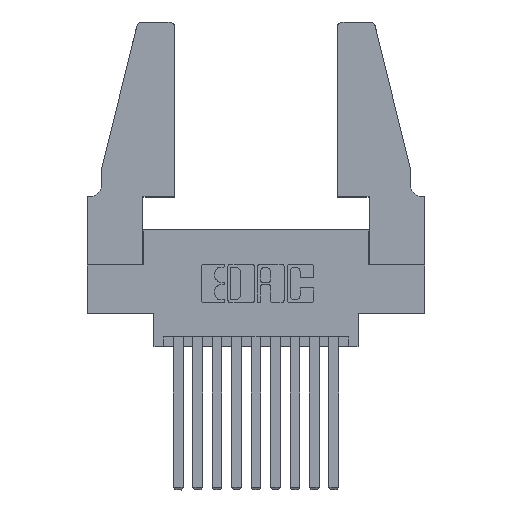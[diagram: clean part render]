
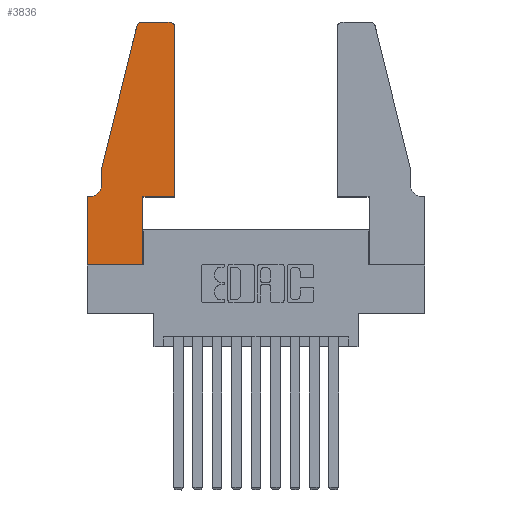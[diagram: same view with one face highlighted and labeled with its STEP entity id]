
A CAD part, top view. The second image highlights one B-rep face of the part: STEP entity #3836.
In plain terms, the highlighted planar face has unit normal (0, 0, 1).
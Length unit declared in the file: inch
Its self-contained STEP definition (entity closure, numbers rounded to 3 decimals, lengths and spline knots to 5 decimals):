
#142 = ORIENTED_EDGE ( 'NONE', *, *, #3117, .T. ) ;
#378 = CARTESIAN_POINT ( 'NONE',  ( 0.0755, 0.5, 0.37 ) ) ;
#531 = DIRECTION ( 'NONE',  ( 1., 0., 0. ) ) ;
#724 = CARTESIAN_POINT ( 'NONE',  ( 0.284, 1.22, 0.37 ) ) ;
#801 = CARTESIAN_POINT ( 'NONE',  ( 0.2865, 0., 0.37 ) ) ;
#998 = VERTEX_POINT ( 'NONE', #2127 ) ;
#1622 = CARTESIAN_POINT ( 'NONE',  ( 0., 0., 0.37 ) ) ;
#1964 = DIRECTION ( 'NONE',  ( 1., 0., 0. ) ) ;
#2127 = CARTESIAN_POINT ( 'NONE',  ( 0.0055, 0.35, 0.37 ) ) ;
#2150 = VECTOR ( 'NONE', #11983, 39.37008 ) ;
#2352 = VECTOR ( 'NONE', #7119, 39.37008 ) ;
#2462 = EDGE_CURVE ( 'NONE', #7469, #9558, #7112, .T. ) ;
#2467 = CARTESIAN_POINT ( 'NONE',  ( 0.0755, 0.42, 0.37 ) ) ;
#2521 = CARTESIAN_POINT ( 'NONE',  ( 0.4505, 0.35, 0.37 ) ) ;
#2615 = CARTESIAN_POINT ( 'NONE',  ( 0.0055, 0.42, 0.37 ) ) ;
#2662 = EDGE_CURVE ( 'NONE', #998, #8964, #7276, .T. ) ;
#2743 = VECTOR ( 'NONE', #531, 39.37008 ) ;
#3000 = CARTESIAN_POINT ( 'NONE',  ( 0.0755, 0.35, 0.37 ) ) ;
#3040 = EDGE_CURVE ( 'NONE', #6112, #5280, #10058, .T. ) ;
#3114 = VERTEX_POINT ( 'NONE', #11042 ) ;
#3117 = EDGE_CURVE ( 'NONE', #9447, #6112, #5302, .T. ) ;
#3128 = PLANE ( 'NONE',  #5755 ) ;
#3197 = CIRCLE ( 'NONE', #11663, 0.03 ) ;
#3413 = ORIENTED_EDGE ( 'NONE', *, *, #12349, .T. ) ;
#3420 = CARTESIAN_POINT ( 'NONE',  ( 0.25487, 1.22718, 0.37 ) ) ;
#3456 = EDGE_CURVE ( 'NONE', #7956, #3114, #5948, .T. ) ;
#3508 = LINE ( 'NONE', #13477, #2352 ) ;
#3756 = ORIENTED_EDGE ( 'NONE', *, *, #2662, .T. ) ;
#3836 = ADVANCED_FACE ( 'NONE', ( #9694 ), #3128, .T. ) ;
#3910 = CARTESIAN_POINT ( 'NONE',  ( 0.4205, 1.22, 0.37 ) ) ;
#4086 = DIRECTION ( 'NONE',  ( 1., 0., 0. ) ) ;
#4266 = ORIENTED_EDGE ( 'NONE', *, *, #5533, .T. ) ;
#4522 = DIRECTION ( 'NONE',  ( 0., 1., 0. ) ) ;
#4706 = DIRECTION ( 'NONE',  ( -0.239, -0.971, 0. ) ) ;
#4798 = DIRECTION ( 'NONE',  ( 1., 0., 0. ) ) ;
#4810 = DIRECTION ( 'NONE',  ( -1., 0., 0. ) ) ;
#4997 = CARTESIAN_POINT ( 'NONE',  ( 0.4205, 1.25, 0.37 ) ) ;
#5167 = VECTOR ( 'NONE', #4798, 39.37008 ) ;
#5257 = ORIENTED_EDGE ( 'NONE', *, *, #9001, .T. ) ;
#5280 = VERTEX_POINT ( 'NONE', #7840 ) ;
#5297 = ORIENTED_EDGE ( 'NONE', *, *, #13607, .T. ) ;
#5302 = CIRCLE ( 'NONE', #8560, 0.03 ) ;
#5330 = CARTESIAN_POINT ( 'NONE',  ( 0., 0., 0.37 ) ) ;
#5533 = EDGE_CURVE ( 'NONE', #9000, #998, #6215, .T. ) ;
#5755 = AXIS2_PLACEMENT_3D ( 'NONE', #13582, #7220, #1964 ) ;
#5793 = CARTESIAN_POINT ( 'NONE',  ( 0.2605, 1.25, 0.37 ) ) ;
#5948 = LINE ( 'NONE', #12916, #12383 ) ;
#6112 = VERTEX_POINT ( 'NONE', #4997 ) ;
#6160 = LINE ( 'NONE', #10082, #5167 ) ;
#6177 = DIRECTION ( 'NONE',  ( -1., 0., 0. ) ) ;
#6215 = CIRCLE ( 'NONE', #13576, 0.07 ) ;
#6617 = DIRECTION ( 'NONE',  ( 0., 1., 0. ) ) ;
#6628 = VECTOR ( 'NONE', #6617, 39.37008 ) ;
#6929 = DIRECTION ( 'NONE',  ( 0., 0., 1. ) ) ;
#6948 = VECTOR ( 'NONE', #6177, 39.37008 ) ;
#6992 = ORIENTED_EDGE ( 'NONE', *, *, #9131, .T. ) ;
#7057 = DIRECTION ( 'NONE',  ( 0., 0., 1. ) ) ;
#7112 = LINE ( 'NONE', #12272, #12245 ) ;
#7119 = DIRECTION ( 'NONE',  ( 0., -1., 0. ) ) ;
#7133 = LINE ( 'NONE', #2521, #6628 ) ;
#7220 = DIRECTION ( 'NONE',  ( 0., 0., 1. ) ) ;
#7276 = LINE ( 'NONE', #3000, #6948 ) ;
#7469 = VERTEX_POINT ( 'NONE', #3420 ) ;
#7623 = CARTESIAN_POINT ( 'NONE',  ( 0., 0.35, 0.37 ) ) ;
#7840 = CARTESIAN_POINT ( 'NONE',  ( 0.284, 1.25, 0.37 ) ) ;
#7956 = VERTEX_POINT ( 'NONE', #801 ) ;
#8044 = DIRECTION ( 'NONE',  ( 1., 0., 0. ) ) ;
#8560 = AXIS2_PLACEMENT_3D ( 'NONE', #3910, #7057, #4086 ) ;
#8763 = CARTESIAN_POINT ( 'NONE',  ( 0.4505, 1.22, 0.37 ) ) ;
#8964 = VERTEX_POINT ( 'NONE', #7623 ) ;
#9000 = VERTEX_POINT ( 'NONE', #2467 ) ;
#9001 = EDGE_CURVE ( 'NONE', #10812, #9447, #7133, .T. ) ;
#9131 = EDGE_CURVE ( 'NONE', #11963, #7956, #11108, .T. ) ;
#9214 = LINE ( 'NONE', #10716, #2150 ) ;
#9447 = VERTEX_POINT ( 'NONE', #8763 ) ;
#9558 = VERTEX_POINT ( 'NONE', #378 ) ;
#9652 = ORIENTED_EDGE ( 'NONE', *, *, #3456, .T. ) ;
#9694 = FACE_OUTER_BOUND ( 'NONE', #12086, .T. ) ;
#9965 = EDGE_CURVE ( 'NONE', #9558, #9000, #3508, .T. ) ;
#10058 = LINE ( 'NONE', #5793, #10715 ) ;
#10082 = CARTESIAN_POINT ( 'NONE',  ( 0.4505, 0.35, 0.37 ) ) ;
#10479 = ORIENTED_EDGE ( 'NONE', *, *, #2462, .T. ) ;
#10715 = VECTOR ( 'NONE', #4810, 39.37008 ) ;
#10716 = CARTESIAN_POINT ( 'NONE',  ( 0., 0., 0.37 ) ) ;
#10812 = VERTEX_POINT ( 'NONE', #12772 ) ;
#11042 = CARTESIAN_POINT ( 'NONE',  ( 0.2865, 0.35, 0.37 ) ) ;
#11101 = DIRECTION ( 'NONE',  ( 0., 0., -1. ) ) ;
#11108 = LINE ( 'NONE', #5330, #2743 ) ;
#11438 = ORIENTED_EDGE ( 'NONE', *, *, #9965, .T. ) ;
#11663 = AXIS2_PLACEMENT_3D ( 'NONE', #724, #6929, #8044 ) ;
#11803 = ORIENTED_EDGE ( 'NONE', *, *, #11928, .T. ) ;
#11928 = EDGE_CURVE ( 'NONE', #8964, #11963, #9214, .T. ) ;
#11941 = ORIENTED_EDGE ( 'NONE', *, *, #3040, .T. ) ;
#11963 = VERTEX_POINT ( 'NONE', #1622 ) ;
#11983 = DIRECTION ( 'NONE',  ( 0., -1., 0. ) ) ;
#12019 = DIRECTION ( 'NONE',  ( -1., 0., 0. ) ) ;
#12086 = EDGE_LOOP ( 'NONE', ( #11941, #5297, #10479, #11438, #4266, #3756, #11803, #6992, #9652, #3413, #5257, #142 ) ) ;
#12245 = VECTOR ( 'NONE', #4706, 39.37008 ) ;
#12272 = CARTESIAN_POINT ( 'NONE',  ( 0.0755, 0.5, 0.37 ) ) ;
#12349 = EDGE_CURVE ( 'NONE', #3114, #10812, #6160, .T. ) ;
#12383 = VECTOR ( 'NONE', #4522, 39.37008 ) ;
#12772 = CARTESIAN_POINT ( 'NONE',  ( 0.4505, 0.35, 0.37 ) ) ;
#12916 = CARTESIAN_POINT ( 'NONE',  ( 0.2865, 0.35, 0.37 ) ) ;
#13477 = CARTESIAN_POINT ( 'NONE',  ( 0.0755, 0.5, 0.37 ) ) ;
#13576 = AXIS2_PLACEMENT_3D ( 'NONE', #2615, #11101, #12019 ) ;
#13582 = CARTESIAN_POINT ( 'NONE',  ( 0., 0.35, 0.37 ) ) ;
#13607 = EDGE_CURVE ( 'NONE', #5280, #7469, #3197, .T. ) ;
